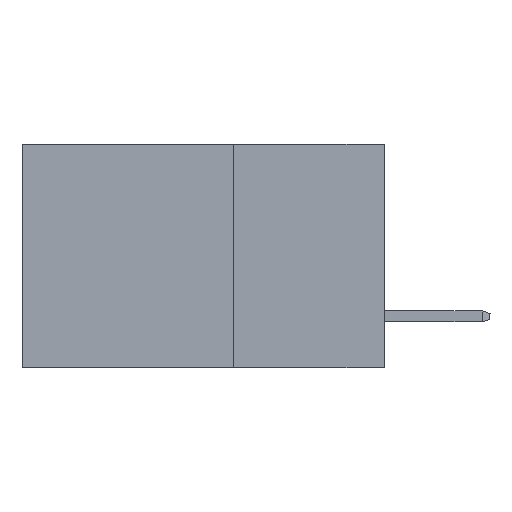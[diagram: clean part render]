
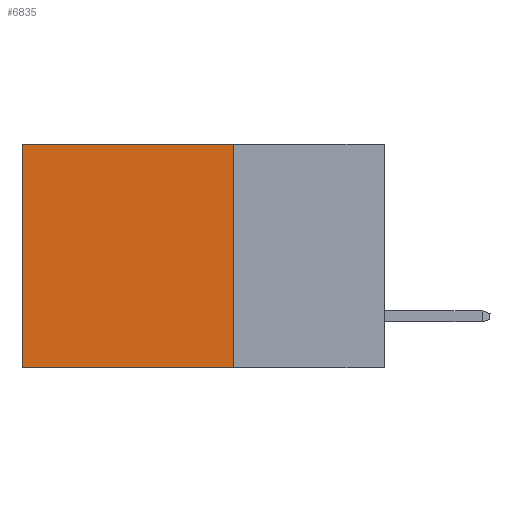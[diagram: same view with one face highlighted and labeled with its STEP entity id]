
A CAD part, left-side view. The second image highlights one B-rep face of the part: STEP entity #6835.
In plain terms, the highlighted planar face has unit normal (-1, 0, 0).
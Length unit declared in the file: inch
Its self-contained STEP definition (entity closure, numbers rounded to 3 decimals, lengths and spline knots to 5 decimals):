
#703 = FACE_OUTER_BOUND ( 'NONE', #8025, .T. ) ;
#805 = LINE ( 'NONE', #7956, #5701 ) ;
#1123 = ORIENTED_EDGE ( 'NONE', *, *, #6455, .F. ) ;
#2023 = VERTEX_POINT ( 'NONE', #12808 ) ;
#2364 = LINE ( 'NONE', #2488, #4340 ) ;
#2488 = CARTESIAN_POINT ( 'NONE',  ( 0.2615, 0.25, -0.37 ) ) ;
#2529 = PLANE ( 'NONE',  #10069 ) ;
#2647 = ORIENTED_EDGE ( 'NONE', *, *, #8617, .T. ) ;
#2766 = CARTESIAN_POINT ( 'NONE',  ( 0.2615, 0.25, 0. ) ) ;
#2980 = VECTOR ( 'NONE', #7346, 39.37008 ) ;
#3095 = DIRECTION ( 'NONE',  ( 0., 0., -1. ) ) ;
#3547 = DIRECTION ( 'NONE',  ( 0., 0., -1. ) ) ;
#4340 = VECTOR ( 'NONE', #3547, 39.37008 ) ;
#4442 = DIRECTION ( 'NONE',  ( 0., 0., -1. ) ) ;
#5701 = VECTOR ( 'NONE', #3095, 39.37008 ) ;
#6232 = CARTESIAN_POINT ( 'NONE',  ( 0.2615, 0.25, 0. ) ) ;
#6362 = LINE ( 'NONE', #6232, #2980 ) ;
#6455 = EDGE_CURVE ( 'NONE', #10259, #12034, #2364, .T. ) ;
#6835 = ADVANCED_FACE ( 'NONE', ( #703 ), #2529, .F. ) ;
#6978 = CARTESIAN_POINT ( 'NONE',  ( 0.2615, 0.25, -0.37 ) ) ;
#7346 = DIRECTION ( 'NONE',  ( 0., 1., 0. ) ) ;
#7659 = CARTESIAN_POINT ( 'NONE',  ( 0.2615, 0.25, -0.37 ) ) ;
#7956 = CARTESIAN_POINT ( 'NONE',  ( 0.2615, 0.6, -0.37 ) ) ;
#7979 = VECTOR ( 'NONE', #10845, 39.37008 ) ;
#8025 = EDGE_LOOP ( 'NONE', ( #2647, #9957, #1123, #8390 ) ) ;
#8390 = ORIENTED_EDGE ( 'NONE', *, *, #11884, .T. ) ;
#8617 = EDGE_CURVE ( 'NONE', #9015, #2023, #805, .T. ) ;
#9015 = VERTEX_POINT ( 'NONE', #12728 ) ;
#9957 = ORIENTED_EDGE ( 'NONE', *, *, #10394, .F. ) ;
#10045 = LINE ( 'NONE', #6978, #7979 ) ;
#10069 = AXIS2_PLACEMENT_3D ( 'NONE', #7659, #11657, #4442 ) ;
#10259 = VERTEX_POINT ( 'NONE', #2766 ) ;
#10394 = EDGE_CURVE ( 'NONE', #12034, #2023, #10045, .T. ) ;
#10845 = DIRECTION ( 'NONE',  ( 0., 1., 0. ) ) ;
#11657 = DIRECTION ( 'NONE',  ( 1., 0., 0. ) ) ;
#11676 = CARTESIAN_POINT ( 'NONE',  ( 0.2615, 0.25, -0.37 ) ) ;
#11884 = EDGE_CURVE ( 'NONE', #10259, #9015, #6362, .T. ) ;
#12034 = VERTEX_POINT ( 'NONE', #11676 ) ;
#12728 = CARTESIAN_POINT ( 'NONE',  ( 0.2615, 0.6, 0. ) ) ;
#12808 = CARTESIAN_POINT ( 'NONE',  ( 0.2615, 0.6, -0.37 ) ) ;
